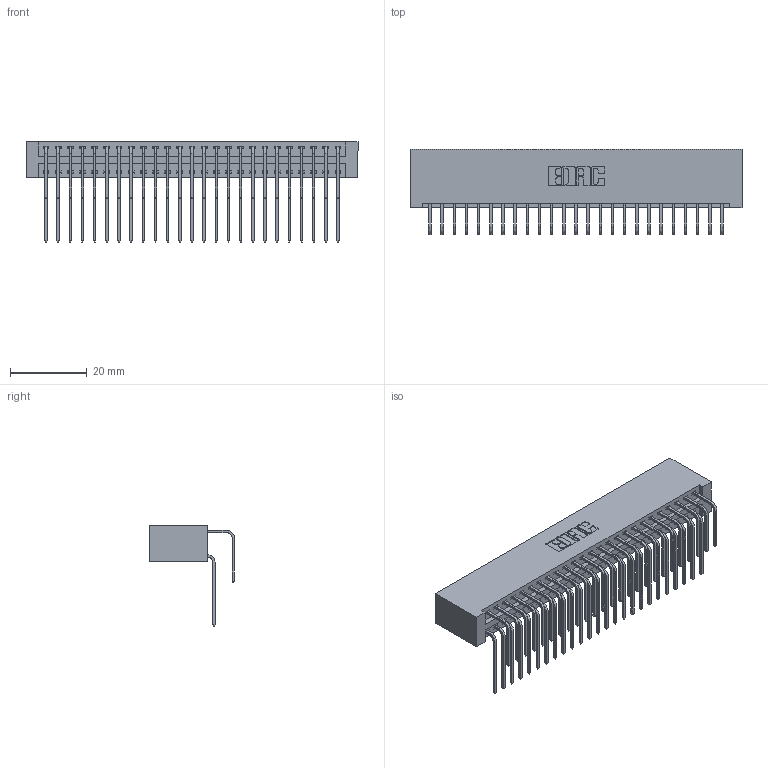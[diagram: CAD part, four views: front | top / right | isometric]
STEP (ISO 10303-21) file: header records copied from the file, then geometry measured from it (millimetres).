
FILE_DESCRIPTION (( 'STEP AP203' ), '1' );
FILE_NAME ('346-050-558-201.STEP', '2018-08-27T22:47:03', ( '' ), ( '' ), 'SwSTEP 2.0', 'SolidWorks 2016', '' );
FILE_SCHEMA (( 'CONFIG_CONTROL_DESIGN' ));
Length unit declared in the file: inch
Products named in the file (4): 346 Part_No Mounting Lugs; 345-292-001_558 559 Tail - 1; 345-292-001_558 Tail - 2; 346-050-558-201
Assembly tree (51 placements, depth 2):
  346-050-558-201
    346 Part_No Mounting Lugs
    345-292-001_558 559 Tail - 1  x25
    345-292-001_558 Tail - 2  x25
Bounding box: 86.61 x 22.16 x 26.16 mm (x, y, z)
Volume: 9175.6 mm3; surface area: 13892.2 mm2
Topology: 51 solids, 51 shells, 2814 faces, 8355 edges, 5502 vertices
Faces by surface type: plane 1922, cylinder 892
Entity records: 20111 total; most frequent: CARTESIAN_POINT 3387, ORIENTED_EDGE 3270, DIRECTION 3003, EDGE_CURVE 1635, LINE 1371, VECTOR 1371, VERTEX_POINT 1086, AXIS2_PLACEMENT_3D 816
